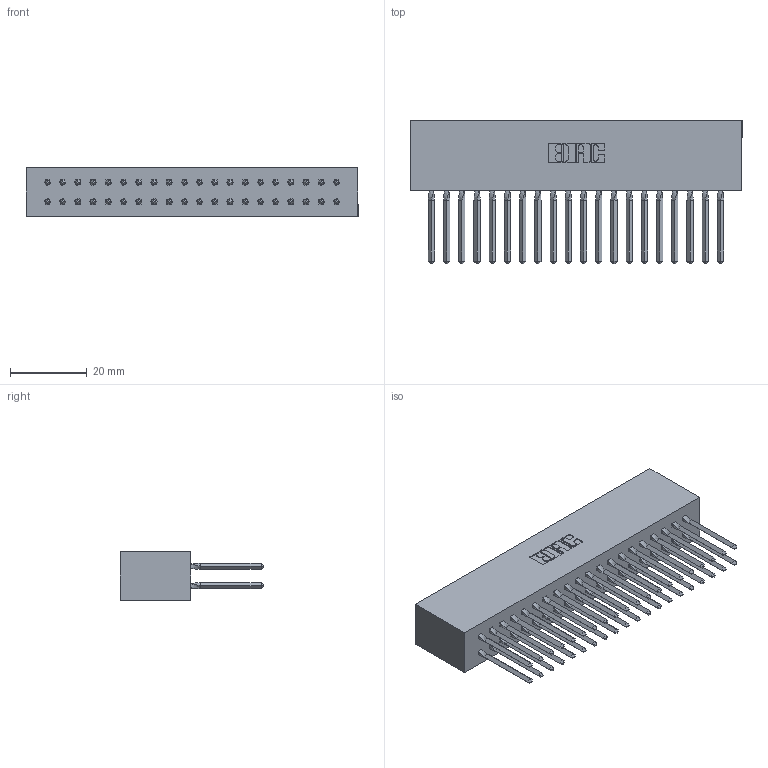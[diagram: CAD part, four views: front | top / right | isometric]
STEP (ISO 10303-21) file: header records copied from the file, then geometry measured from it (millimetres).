
FILE_DESCRIPTION (( 'STEP AP203' ), '1' );
FILE_NAME ('317-040-540-801.STEP', '2020-02-28T00:25:06', ( '' ), ( '' ), 'SwSTEP 2.0', 'SolidWorks 2016', '' );
FILE_SCHEMA (( 'CONFIG_CONTROL_DESIGN' ));
Length unit declared in the file: inch
Products named in the file (3): 317-290-001_540; 317-040-540-801; 317 Part_Lugless
Assembly tree (41 placements, depth 2):
  317-040-540-801
    317 Part_Lugless
    317-290-001_540  x40
Bounding box: 86.46 x 37.34 x 12.7 mm (x, y, z)
Volume: 15560.7 mm3; surface area: 22625.3 mm2
Topology: 41 solids, 41 shells, 3650 faces, 10119 edges, 6518 vertices
Faces by surface type: plane 2970, cylinder 520, bspline 160
Entity records: 31570 total; most frequent: CARTESIAN_POINT 5919, ORIENTED_EDGE 5418, DIRECTION 4515, EDGE_CURVE 2709, LINE 2461, VECTOR 2461, VERTEX_POINT 1799, AXIS2_PLACEMENT_3D 1027
